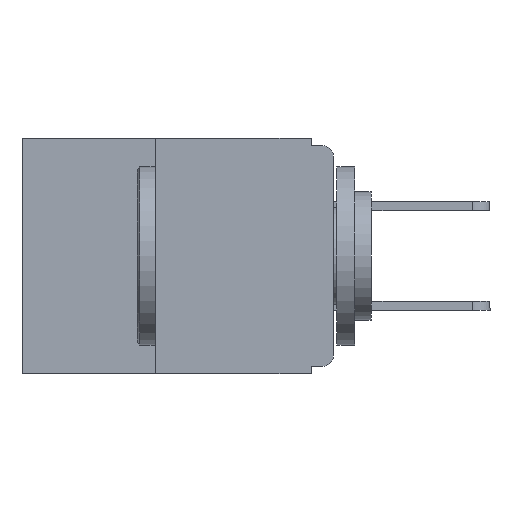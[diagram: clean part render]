
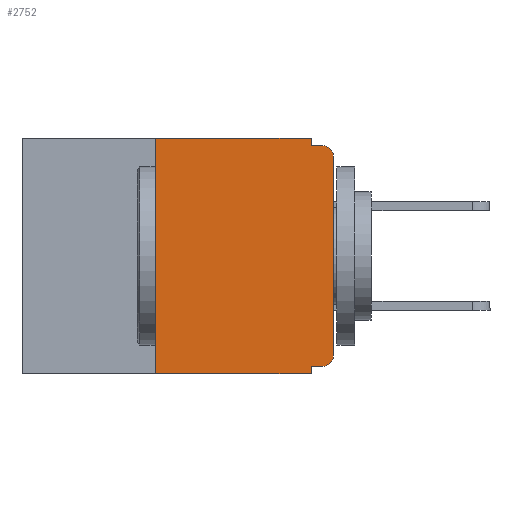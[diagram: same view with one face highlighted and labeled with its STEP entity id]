
A CAD part, left-side view. The second image highlights one B-rep face of the part: STEP entity #2752.
In plain terms, the highlighted planar face has unit normal (-1, 0, 0).
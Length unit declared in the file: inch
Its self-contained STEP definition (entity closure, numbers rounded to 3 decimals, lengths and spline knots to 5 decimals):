
#302 = CARTESIAN_POINT ( 'NONE',  ( 0., 0.031, -0.01 ) ) ;
#410 = CARTESIAN_POINT ( 'NONE',  ( 0., 0.25, 0. ) ) ;
#648 = DIRECTION ( 'NONE',  ( 0., -1., 0. ) ) ;
#1367 = EDGE_CURVE ( 'NONE', #18277, #2247, #19449, .T. ) ;
#1543 = EDGE_CURVE ( 'NONE', #8382, #11193, #13021, .T. ) ;
#1917 = CARTESIAN_POINT ( 'NONE',  ( 0., 0., -0.025 ) ) ;
#1943 = EDGE_CURVE ( 'NONE', #2772, #3808, #18529, .T. ) ;
#2058 = ORIENTED_EDGE ( 'NONE', *, *, #12156, .T. ) ;
#2247 = VERTEX_POINT ( 'NONE', #15820 ) ;
#2418 = LINE ( 'NONE', #8059, #14798 ) ;
#2524 = EDGE_CURVE ( 'NONE', #12954, #2247, #9280, .T. ) ;
#2699 = DIRECTION ( 'NONE',  ( 0., 0., -1. ) ) ;
#2752 = ADVANCED_FACE ( 'NONE', ( #9013 ), #8290, .F. ) ;
#2772 = VERTEX_POINT ( 'NONE', #410 ) ;
#2907 = DIRECTION ( 'NONE',  ( 0., 0., -1. ) ) ;
#2948 = ORIENTED_EDGE ( 'NONE', *, *, #8271, .T. ) ;
#2970 = DIRECTION ( 'NONE',  ( 1., 0., 0. ) ) ;
#3486 = LINE ( 'NONE', #11462, #19770 ) ;
#3808 = VERTEX_POINT ( 'NONE', #15799 ) ;
#4217 = ORIENTED_EDGE ( 'NONE', *, *, #17720, .F. ) ;
#4726 = ORIENTED_EDGE ( 'NONE', *, *, #7041, .F. ) ;
#5148 = ORIENTED_EDGE ( 'NONE', *, *, #1943, .F. ) ;
#5214 = ORIENTED_EDGE ( 'NONE', *, *, #5949, .F. ) ;
#5438 = ORIENTED_EDGE ( 'NONE', *, *, #2524, .T. ) ;
#5871 = VECTOR ( 'NONE', #11123, 39.37008 ) ;
#5949 = EDGE_CURVE ( 'NONE', #12954, #2772, #19310, .T. ) ;
#6434 = ORIENTED_EDGE ( 'NONE', *, *, #1367, .F. ) ;
#7021 = ORIENTED_EDGE ( 'NONE', *, *, #11498, .F. ) ;
#7041 = EDGE_CURVE ( 'NONE', #3808, #9297, #9376, .T. ) ;
#7109 = CARTESIAN_POINT ( 'NONE',  ( 0., 0., -0.305 ) ) ;
#7232 = ORIENTED_EDGE ( 'NONE', *, *, #1543, .T. ) ;
#7304 = DIRECTION ( 'NONE',  ( 0., -1., 0. ) ) ;
#7558 = VECTOR ( 'NONE', #2699, 39.37008 ) ;
#7892 = CARTESIAN_POINT ( 'NONE',  ( 0., 0.437, 0. ) ) ;
#7985 = CARTESIAN_POINT ( 'NONE',  ( 0., 0.437, 0. ) ) ;
#8059 = CARTESIAN_POINT ( 'NONE',  ( 0., 0., 0. ) ) ;
#8271 = EDGE_CURVE ( 'NONE', #9219, #19566, #17387, .T. ) ;
#8290 = PLANE ( 'NONE',  #14562 ) ;
#8382 = VERTEX_POINT ( 'NONE', #11505 ) ;
#8790 = VECTOR ( 'NONE', #7304, 39.37008 ) ;
#8796 = AXIS2_PLACEMENT_3D ( 'NONE', #14191, #13141, #20332 ) ;
#8954 = CARTESIAN_POINT ( 'NONE',  ( 0., 0.25, -0.33 ) ) ;
#9013 = FACE_OUTER_BOUND ( 'NONE', #16770, .T. ) ;
#9219 = VERTEX_POINT ( 'NONE', #1917 ) ;
#9280 = LINE ( 'NONE', #16733, #8790 ) ;
#9297 = VERTEX_POINT ( 'NONE', #302 ) ;
#9376 = LINE ( 'NONE', #16205, #9878 ) ;
#9878 = VECTOR ( 'NONE', #16526, 39.37008 ) ;
#10194 = LINE ( 'NONE', #18776, #5871 ) ;
#10318 = VECTOR ( 'NONE', #648, 39.37008 ) ;
#10357 = AXIS2_PLACEMENT_3D ( 'NONE', #12628, #12611, #12593 ) ;
#10367 = DIRECTION ( 'NONE',  ( 0., 0., 1. ) ) ;
#10392 = CARTESIAN_POINT ( 'NONE',  ( 0., 0.25, -0.33 ) ) ;
#10770 = CARTESIAN_POINT ( 'NONE',  ( 0., 0.015, -0.01 ) ) ;
#11123 = DIRECTION ( 'NONE',  ( 0., 1., 0. ) ) ;
#11193 = VERTEX_POINT ( 'NONE', #7109 ) ;
#11462 = CARTESIAN_POINT ( 'NONE',  ( 0., 0., -0.01 ) ) ;
#11498 = EDGE_CURVE ( 'NONE', #8382, #18277, #10194, .T. ) ;
#11505 = CARTESIAN_POINT ( 'NONE',  ( 0., 0.015, -0.32 ) ) ;
#12147 = VECTOR ( 'NONE', #10367, 39.37008 ) ;
#12156 = EDGE_CURVE ( 'NONE', #11193, #9219, #2418, .T. ) ;
#12593 = DIRECTION ( 'NONE',  ( 0., 0., -1. ) ) ;
#12611 = DIRECTION ( 'NONE',  ( -1., 0., 0. ) ) ;
#12628 = CARTESIAN_POINT ( 'NONE',  ( 0., 0.015, -0.025 ) ) ;
#12954 = VERTEX_POINT ( 'NONE', #8954 ) ;
#13021 = CIRCLE ( 'NONE', #8796, 0.015 ) ;
#13141 = DIRECTION ( 'NONE',  ( -1., 0., 0. ) ) ;
#14191 = CARTESIAN_POINT ( 'NONE',  ( 0., 0.015, -0.305 ) ) ;
#14562 = AXIS2_PLACEMENT_3D ( 'NONE', #7892, #2970, #2907 ) ;
#14798 = VECTOR ( 'NONE', #17458, 39.37008 ) ;
#15799 = CARTESIAN_POINT ( 'NONE',  ( 0., 0.031, 0. ) ) ;
#15820 = CARTESIAN_POINT ( 'NONE',  ( 0., 0.031, -0.33 ) ) ;
#16205 = CARTESIAN_POINT ( 'NONE',  ( 0., 0.031, 0. ) ) ;
#16526 = DIRECTION ( 'NONE',  ( 0., 0., -1. ) ) ;
#16733 = CARTESIAN_POINT ( 'NONE',  ( 0., 0.437, -0.33 ) ) ;
#16770 = EDGE_LOOP ( 'NONE', ( #2058, #2948, #4217, #4726, #5148, #5214, #5438, #6434, #7021, #7232 ) ) ;
#17387 = CIRCLE ( 'NONE', #10357, 0.015 ) ;
#17458 = DIRECTION ( 'NONE',  ( 0., 0., 1. ) ) ;
#17684 = DIRECTION ( 'NONE',  ( 0., -1., 0. ) ) ;
#17720 = EDGE_CURVE ( 'NONE', #9297, #19566, #3486, .T. ) ;
#18090 = CARTESIAN_POINT ( 'NONE',  ( 0., 0.031, -0.33 ) ) ;
#18277 = VERTEX_POINT ( 'NONE', #20569 ) ;
#18529 = LINE ( 'NONE', #7985, #10318 ) ;
#18776 = CARTESIAN_POINT ( 'NONE',  ( 0., 0., -0.32 ) ) ;
#19310 = LINE ( 'NONE', #10392, #12147 ) ;
#19449 = LINE ( 'NONE', #18090, #7558 ) ;
#19566 = VERTEX_POINT ( 'NONE', #10770 ) ;
#19770 = VECTOR ( 'NONE', #17684, 39.37008 ) ;
#20332 = DIRECTION ( 'NONE',  ( 0., 0., -1. ) ) ;
#20569 = CARTESIAN_POINT ( 'NONE',  ( 0., 0.031, -0.32 ) ) ;
